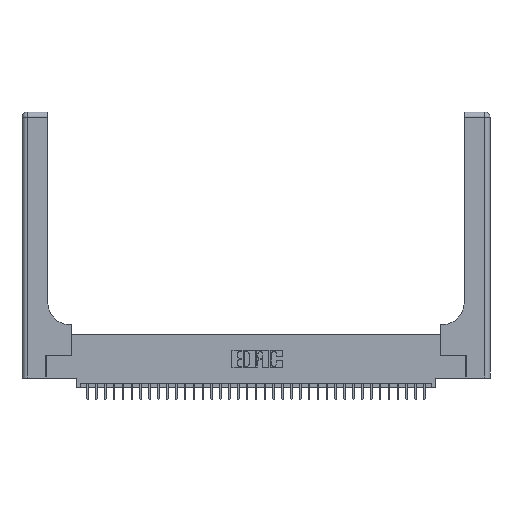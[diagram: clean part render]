
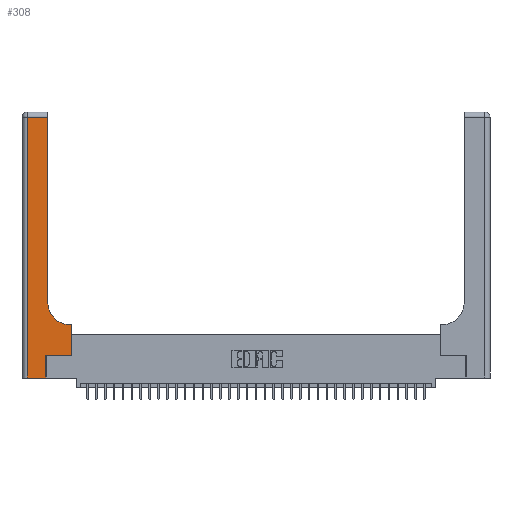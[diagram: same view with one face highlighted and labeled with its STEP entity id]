
A CAD part, top view. The second image highlights one B-rep face of the part: STEP entity #308.
In plain terms, the highlighted planar face has unit normal (0, 0, 1).
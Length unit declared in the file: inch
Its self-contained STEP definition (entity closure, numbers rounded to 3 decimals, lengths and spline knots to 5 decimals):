
#308 = ADVANCED_FACE ( 'NONE', ( #33484 ), #5806, .F. ) ;
#351 = LINE ( 'NONE', #16941, #8172 ) ;
#2087 = LINE ( 'NONE', #6894, #11641 ) ;
#2244 = VECTOR ( 'NONE', #8124, 39.37008 ) ;
#2261 = CARTESIAN_POINT ( 'NONE',  ( 0.269, 0., 0.37 ) ) ;
#2581 = AXIS2_PLACEMENT_3D ( 'NONE', #22275, #5672, #36282 ) ;
#2593 = VECTOR ( 'NONE', #11850, 39.37008 ) ;
#2767 = CARTESIAN_POINT ( 'NONE',  ( 0.5415, 0.6, 0.37 ) ) ;
#3074 = EDGE_LOOP ( 'NONE', ( #17838, #18434, #30754, #14331, #5573, #13638, #16224, #4992, #20615 ) ) ;
#4657 = DIRECTION ( 'NONE',  ( -1., 0., 0. ) ) ;
#4992 = ORIENTED_EDGE ( 'NONE', *, *, #29264, .T. ) ;
#5391 = VERTEX_POINT ( 'NONE', #6788 ) ;
#5573 = ORIENTED_EDGE ( 'NONE', *, *, #28705, .T. ) ;
#5662 = DIRECTION ( 'NONE',  ( 1., 0., 0. ) ) ;
#5672 = DIRECTION ( 'NONE',  ( 0., 0., -1. ) ) ;
#5806 = PLANE ( 'NONE',  #13015 ) ;
#6738 = CARTESIAN_POINT ( 'NONE',  ( 0.269, 0., 0.37 ) ) ;
#6788 = CARTESIAN_POINT ( 'NONE',  ( 0.269, 0.25, 0.37 ) ) ;
#6894 = CARTESIAN_POINT ( 'NONE',  ( 0., 2.94, 0.37 ) ) ;
#8124 = DIRECTION ( 'NONE',  ( 0., -1., 0. ) ) ;
#8172 = VECTOR ( 'NONE', #4657, 39.37008 ) ;
#8602 = LINE ( 'NONE', #17623, #20883 ) ;
#11027 = EDGE_CURVE ( 'NONE', #18801, #19437, #30031, .T. ) ;
#11093 = VECTOR ( 'NONE', #11110, 39.37008 ) ;
#11110 = DIRECTION ( 'NONE',  ( 0., 1., 0. ) ) ;
#11233 = VECTOR ( 'NONE', #12719, 39.37008 ) ;
#11346 = DIRECTION ( 'NONE',  ( -1., 0., 0. ) ) ;
#11641 = VECTOR ( 'NONE', #24574, 39.37008 ) ;
#11760 = VERTEX_POINT ( 'NONE', #6738 ) ;
#11850 = DIRECTION ( 'NONE',  ( 0., 1., 0. ) ) ;
#12719 = DIRECTION ( 'NONE',  ( 0., 1., 0. ) ) ;
#13015 = AXIS2_PLACEMENT_3D ( 'NONE', #30697, #19633, #11346 ) ;
#13265 = CARTESIAN_POINT ( 'NONE',  ( 0.5585, 0.25, 0.37 ) ) ;
#13638 = ORIENTED_EDGE ( 'NONE', *, *, #26696, .T. ) ;
#14331 = ORIENTED_EDGE ( 'NONE', *, *, #36349, .T. ) ;
#14600 = LINE ( 'NONE', #25838, #2593 ) ;
#16224 = ORIENTED_EDGE ( 'NONE', *, *, #11027, .T. ) ;
#16600 = CARTESIAN_POINT ( 'NONE',  ( 0.06, 3., 0.37 ) ) ;
#16941 = CARTESIAN_POINT ( 'NONE',  ( 0.2915, 0.6, 0.37 ) ) ;
#17170 = EDGE_CURVE ( 'NONE', #30300, #19205, #21410, .T. ) ;
#17623 = CARTESIAN_POINT ( 'NONE',  ( 0., 0., 0.37 ) ) ;
#17838 = ORIENTED_EDGE ( 'NONE', *, *, #21934, .T. ) ;
#18163 = VERTEX_POINT ( 'NONE', #18427 ) ;
#18427 = CARTESIAN_POINT ( 'NONE',  ( 0.06, 0., 0.37 ) ) ;
#18434 = ORIENTED_EDGE ( 'NONE', *, *, #29861, .T. ) ;
#18801 = VERTEX_POINT ( 'NONE', #23188 ) ;
#19134 = LINE ( 'NONE', #30914, #27441 ) ;
#19205 = VERTEX_POINT ( 'NONE', #20366 ) ;
#19361 = LINE ( 'NONE', #16600, #2244 ) ;
#19437 = VERTEX_POINT ( 'NONE', #27892 ) ;
#19633 = DIRECTION ( 'NONE',  ( 0., 0., -1. ) ) ;
#20366 = CARTESIAN_POINT ( 'NONE',  ( 0.2915, 0.85, 0.37 ) ) ;
#20615 = ORIENTED_EDGE ( 'NONE', *, *, #17170, .T. ) ;
#20883 = VECTOR ( 'NONE', #28855, 39.37008 ) ;
#21410 = CIRCLE ( 'NONE', #2581, 0.25 ) ;
#21934 = EDGE_CURVE ( 'NONE', #19205, #29272, #14600, .T. ) ;
#22275 = CARTESIAN_POINT ( 'NONE',  ( 0.5415, 0.85, 0.37 ) ) ;
#23188 = CARTESIAN_POINT ( 'NONE',  ( 0.5585, 0.25, 0.37 ) ) ;
#23259 = VERTEX_POINT ( 'NONE', #30064 ) ;
#24574 = DIRECTION ( 'NONE',  ( -1., 0., 0. ) ) ;
#25838 = CARTESIAN_POINT ( 'NONE',  ( 0.2915, 3., 0.37 ) ) ;
#26696 = EDGE_CURVE ( 'NONE', #5391, #18801, #19134, .T. ) ;
#27441 = VECTOR ( 'NONE', #5662, 39.37008 ) ;
#27892 = CARTESIAN_POINT ( 'NONE',  ( 0.5585, 0.6, 0.37 ) ) ;
#28189 = CARTESIAN_POINT ( 'NONE',  ( 0.2915, 2.94, 0.37 ) ) ;
#28705 = EDGE_CURVE ( 'NONE', #11760, #5391, #33239, .T. ) ;
#28855 = DIRECTION ( 'NONE',  ( 1., 0., 0. ) ) ;
#29264 = EDGE_CURVE ( 'NONE', #19437, #30300, #351, .T. ) ;
#29272 = VERTEX_POINT ( 'NONE', #28189 ) ;
#29861 = EDGE_CURVE ( 'NONE', #29272, #23259, #2087, .T. ) ;
#30031 = LINE ( 'NONE', #13265, #11233 ) ;
#30064 = CARTESIAN_POINT ( 'NONE',  ( 0.06, 2.94, 0.37 ) ) ;
#30300 = VERTEX_POINT ( 'NONE', #2767 ) ;
#30308 = EDGE_CURVE ( 'NONE', #23259, #18163, #19361, .T. ) ;
#30697 = CARTESIAN_POINT ( 'NONE',  ( 0., 3., 0.37 ) ) ;
#30754 = ORIENTED_EDGE ( 'NONE', *, *, #30308, .T. ) ;
#30914 = CARTESIAN_POINT ( 'NONE',  ( 0.269, 0.25, 0.37 ) ) ;
#33239 = LINE ( 'NONE', #2261, #11093 ) ;
#33484 = FACE_OUTER_BOUND ( 'NONE', #3074, .T. ) ;
#36282 = DIRECTION ( 'NONE',  ( 1., 0., 0. ) ) ;
#36349 = EDGE_CURVE ( 'NONE', #18163, #11760, #8602, .T. ) ;
